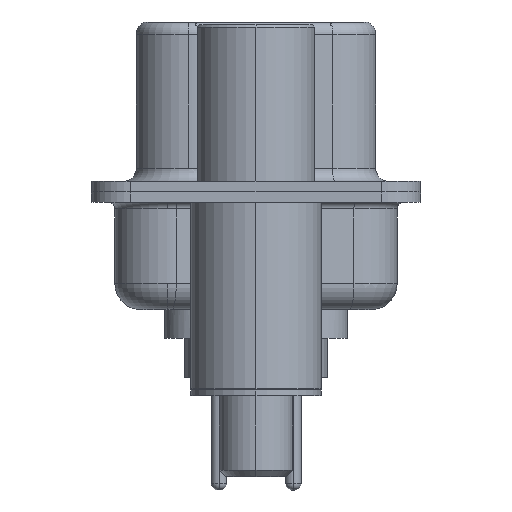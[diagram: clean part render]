
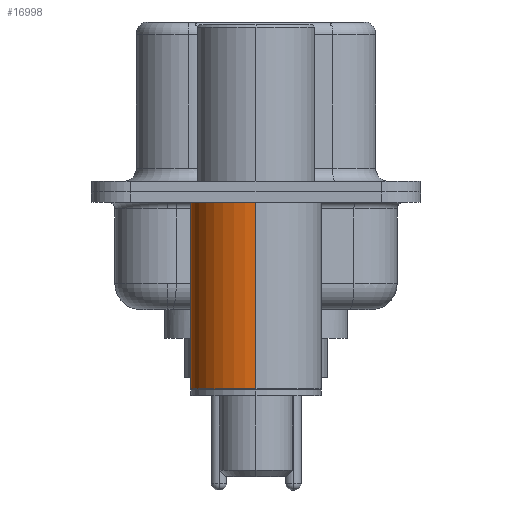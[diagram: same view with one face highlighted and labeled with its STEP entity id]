
A CAD part, left-side view. The second image highlights one B-rep face of the part: STEP entity #16998.
In plain terms, the highlighted cylindrical face has radius 2.5 mm (diameter 5 mm), a partial arc.
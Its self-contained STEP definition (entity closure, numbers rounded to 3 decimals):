
#20 = CIRCLE ( 'NONE', #5414, 2.5 ) ;
#60 = VECTOR ( 'NONE', #13155, 1000. ) ;
#333 = CYLINDRICAL_SURFACE ( 'NONE', #9750, 2.5 ) ;
#2155 = VECTOR ( 'NONE', #6487, 1000. ) ;
#3925 = ORIENTED_EDGE ( 'NONE', *, *, #16738, .F. ) ;
#4910 = DIRECTION ( 'NONE',  ( 0., 0., 1. ) ) ;
#5244 = DIRECTION ( 'NONE',  ( 0., 0., 1. ) ) ;
#5414 = AXIS2_PLACEMENT_3D ( 'NONE', #19882, #9202, #21735 ) ;
#6487 = DIRECTION ( 'NONE',  ( 0., 0., 1. ) ) ;
#7871 = EDGE_CURVE ( 'NONE', #20978, #14519, #20, .T. ) ;
#8069 = CARTESIAN_POINT ( 'NONE',  ( 2.5, 0., -0.4 ) ) ;
#8474 = CARTESIAN_POINT ( 'NONE',  ( 0., 0., 0.581 ) ) ;
#9202 = DIRECTION ( 'NONE',  ( 0., 0., 1. ) ) ;
#9750 = AXIS2_PLACEMENT_3D ( 'NONE', #8474, #4910, #12164 ) ;
#10626 = CARTESIAN_POINT ( 'NONE',  ( 2.5, 0., -7.525 ) ) ;
#11401 = CARTESIAN_POINT ( 'NONE',  ( 2.5, 0., 0.581 ) ) ;
#12164 = DIRECTION ( 'NONE',  ( 1., 0., 0. ) ) ;
#13155 = DIRECTION ( 'NONE',  ( 0., 0., 1. ) ) ;
#13166 = ORIENTED_EDGE ( 'NONE', *, *, #23408, .F. ) ;
#13591 = EDGE_CURVE ( 'NONE', #14519, #22818, #20768, .T. ) ;
#14506 = LINE ( 'NONE', #11401, #60 ) ;
#14519 = VERTEX_POINT ( 'NONE', #16235 ) ;
#14766 = FACE_OUTER_BOUND ( 'NONE', #18512, .T. ) ;
#15017 = CIRCLE ( 'NONE', #21246, 2.5 ) ;
#15418 = CARTESIAN_POINT ( 'NONE',  ( -2.5, 0., 0.581 ) ) ;
#15987 = CARTESIAN_POINT ( 'NONE',  ( 0., 0., -0.4 ) ) ;
#16235 = CARTESIAN_POINT ( 'NONE',  ( -2.5, 0., -7.525 ) ) ;
#16738 = EDGE_CURVE ( 'NONE', #20978, #21932, #14506, .T. ) ;
#16998 = ADVANCED_FACE ( 'NONE', ( #14766 ), #333, .T. ) ;
#17763 = DIRECTION ( 'NONE',  ( 1., 0., 0. ) ) ;
#18512 = EDGE_LOOP ( 'NONE', ( #22671, #20033, #13166, #3925 ) ) ;
#19882 = CARTESIAN_POINT ( 'NONE',  ( 0., 0., -7.525 ) ) ;
#20033 = ORIENTED_EDGE ( 'NONE', *, *, #13591, .T. ) ;
#20768 = LINE ( 'NONE', #15418, #2155 ) ;
#20978 = VERTEX_POINT ( 'NONE', #10626 ) ;
#21246 = AXIS2_PLACEMENT_3D ( 'NONE', #15987, #5244, #17763 ) ;
#21735 = DIRECTION ( 'NONE',  ( 1., 0., 0. ) ) ;
#21932 = VERTEX_POINT ( 'NONE', #8069 ) ;
#22671 = ORIENTED_EDGE ( 'NONE', *, *, #7871, .T. ) ;
#22818 = VERTEX_POINT ( 'NONE', #23243 ) ;
#23243 = CARTESIAN_POINT ( 'NONE',  ( -2.5, 0., -0.4 ) ) ;
#23408 = EDGE_CURVE ( 'NONE', #21932, #22818, #15017, .T. ) ;
